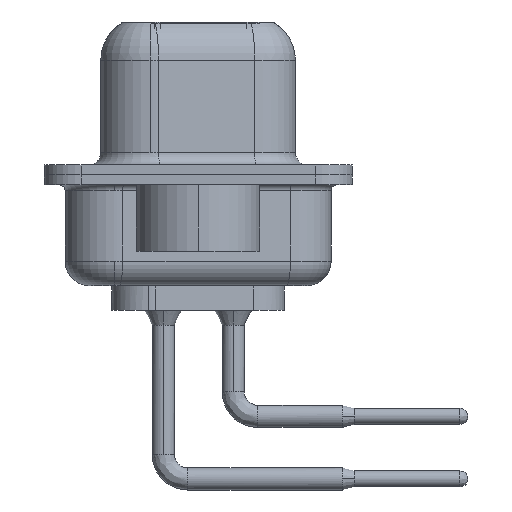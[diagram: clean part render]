
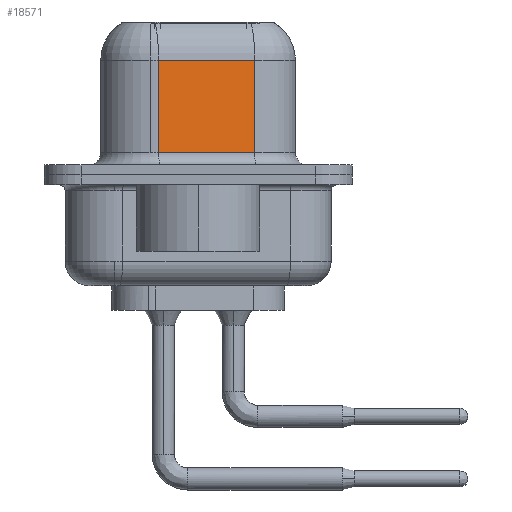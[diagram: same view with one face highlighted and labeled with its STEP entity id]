
A CAD part, left-side view. The second image highlights one B-rep face of the part: STEP entity #18571.
In plain terms, the highlighted planar face has unit normal (-0.985, -0.174, 0).
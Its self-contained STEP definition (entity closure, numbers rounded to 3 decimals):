
#169 = AXIS2_PLACEMENT_3D ( 'NONE', #24903, #8709, #22905 ) ;
#814 = VECTOR ( 'NONE', #17243, 1000. ) ;
#1876 = LINE ( 'NONE', #24878, #18861 ) ;
#3340 = VERTEX_POINT ( 'NONE', #22038 ) ;
#3681 = FACE_OUTER_BOUND ( 'NONE', #4422, .T. ) ;
#4005 = DIRECTION ( 'NONE',  ( 0., 0., -1. ) ) ;
#4422 = EDGE_LOOP ( 'NONE', ( #8413, #24648, #25288, #6100 ) ) ;
#5023 = EDGE_CURVE ( 'NONE', #3340, #24557, #7642, .T. ) ;
#5632 = VERTEX_POINT ( 'NONE', #22961 ) ;
#6100 = ORIENTED_EDGE ( 'NONE', *, *, #9291, .T. ) ;
#6435 = LINE ( 'NONE', #19150, #814 ) ;
#6589 = PLANE ( 'NONE',  #169 ) ;
#7103 = EDGE_CURVE ( 'NONE', #21645, #5632, #11796, .T. ) ;
#7642 = LINE ( 'NONE', #10968, #17789 ) ;
#7732 = CARTESIAN_POINT ( 'NONE',  ( 5.068, -2.297, 0.9 ) ) ;
#8413 = ORIENTED_EDGE ( 'NONE', *, *, #5023, .F. ) ;
#8709 = DIRECTION ( 'NONE',  ( 0.985, 0.174, 0. ) ) ;
#9291 = EDGE_CURVE ( 'NONE', #5632, #24557, #1876, .T. ) ;
#10531 = VECTOR ( 'NONE', #4005, 1000. ) ;
#10968 = CARTESIAN_POINT ( 'NONE',  ( 5.068, -2.297, 6.4 ) ) ;
#11796 = LINE ( 'NONE', #20394, #10531 ) ;
#14987 = DIRECTION ( 'NONE',  ( 0., 0., -1. ) ) ;
#17243 = DIRECTION ( 'NONE',  ( -0.174, 0.985, 0. ) ) ;
#17789 = VECTOR ( 'NONE', #14987, 1000. ) ;
#18571 = ADVANCED_FACE ( 'NONE', ( #3681 ), #6589, .F. ) ;
#18861 = VECTOR ( 'NONE', #20733, 1000. ) ;
#19150 = CARTESIAN_POINT ( 'NONE',  ( 5.068, -2.297, 4.65 ) ) ;
#19292 = EDGE_CURVE ( 'NONE', #3340, #21645, #6435, .T. ) ;
#20394 = CARTESIAN_POINT ( 'NONE',  ( 4.38, 1.603, 6.4 ) ) ;
#20733 = DIRECTION ( 'NONE',  ( 0.174, -0.985, 0. ) ) ;
#21450 = CARTESIAN_POINT ( 'NONE',  ( 4.38, 1.603, 4.65 ) ) ;
#21645 = VERTEX_POINT ( 'NONE', #21450 ) ;
#22038 = CARTESIAN_POINT ( 'NONE',  ( 5.068, -2.297, 4.65 ) ) ;
#22905 = DIRECTION ( 'NONE',  ( -0.174, 0.985, 0. ) ) ;
#22961 = CARTESIAN_POINT ( 'NONE',  ( 4.38, 1.603, 0.9 ) ) ;
#24557 = VERTEX_POINT ( 'NONE', #7732 ) ;
#24648 = ORIENTED_EDGE ( 'NONE', *, *, #19292, .T. ) ;
#24878 = CARTESIAN_POINT ( 'NONE',  ( 5.068, -2.297, 0.9 ) ) ;
#24903 = CARTESIAN_POINT ( 'NONE',  ( 5.068, -2.297, 6.4 ) ) ;
#25288 = ORIENTED_EDGE ( 'NONE', *, *, #7103, .T. ) ;
